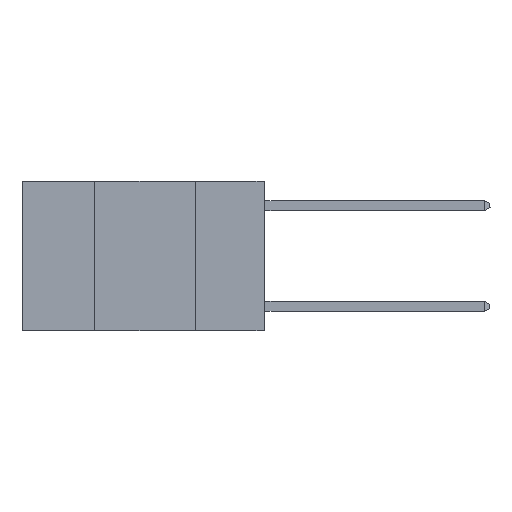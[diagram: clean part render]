
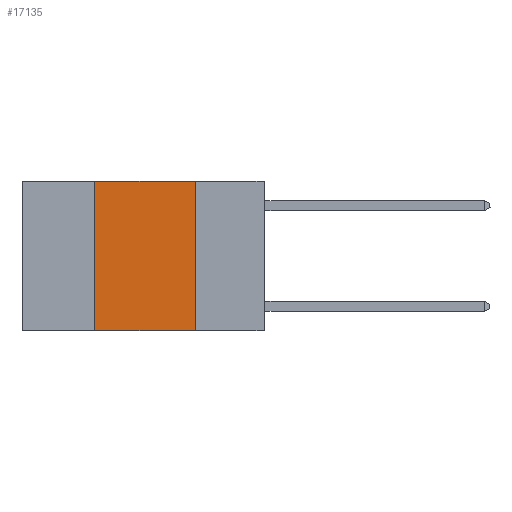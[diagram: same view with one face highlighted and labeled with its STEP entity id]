
A CAD part, left-side view. The second image highlights one B-rep face of the part: STEP entity #17135.
In plain terms, the highlighted planar face has unit normal (-1, 0, 0).
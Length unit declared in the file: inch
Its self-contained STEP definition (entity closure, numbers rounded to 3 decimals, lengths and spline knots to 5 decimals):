
#3728 = VECTOR ( 'NONE', #23854, 39.37008 ) ;
#3889 = LINE ( 'NONE', #4177, #15653 ) ;
#4177 = CARTESIAN_POINT ( 'NONE',  ( 0., 0.17, 0. ) ) ;
#4982 = VECTOR ( 'NONE', #8364, 39.37008 ) ;
#5128 = CARTESIAN_POINT ( 'NONE',  ( 0., 0.6, 0. ) ) ;
#6012 = CARTESIAN_POINT ( 'NONE',  ( 0., 0.6, -0.37 ) ) ;
#6512 = DIRECTION ( 'NONE',  ( 0., 0., -1. ) ) ;
#6677 = CARTESIAN_POINT ( 'NONE',  ( 0., 0.42, 0. ) ) ;
#8065 = DIRECTION ( 'NONE',  ( 1., 0., 0. ) ) ;
#8364 = DIRECTION ( 'NONE',  ( 0., -1., 0. ) ) ;
#8376 = EDGE_LOOP ( 'NONE', ( #15675, #22014, #15089, #15816 ) ) ;
#8590 = DIRECTION ( 'NONE',  ( 0., 0., 1. ) ) ;
#9260 = EDGE_CURVE ( 'NONE', #24364, #10238, #3889, .T. ) ;
#10238 = VERTEX_POINT ( 'NONE', #14322 ) ;
#13587 = EDGE_CURVE ( 'NONE', #28700, #24364, #23144, .T. ) ;
#14322 = CARTESIAN_POINT ( 'NONE',  ( 0., 0.17, -0.37 ) ) ;
#15089 = ORIENTED_EDGE ( 'NONE', *, *, #20933, .F. ) ;
#15090 = CARTESIAN_POINT ( 'NONE',  ( 0., 0.6, 0. ) ) ;
#15246 = LINE ( 'NONE', #17965, #26885 ) ;
#15653 = VECTOR ( 'NONE', #6512, 39.37008 ) ;
#15675 = ORIENTED_EDGE ( 'NONE', *, *, #9260, .F. ) ;
#15816 = ORIENTED_EDGE ( 'NONE', *, *, #25474, .T. ) ;
#16163 = CARTESIAN_POINT ( 'NONE',  ( 0., 0.17, 0. ) ) ;
#16275 = AXIS2_PLACEMENT_3D ( 'NONE', #15090, #8065, #24436 ) ;
#16429 = CARTESIAN_POINT ( 'NONE',  ( 0., 0.42, -0.37 ) ) ;
#16813 = VERTEX_POINT ( 'NONE', #16429 ) ;
#17135 = ADVANCED_FACE ( 'NONE', ( #17694 ), #19806, .F. ) ;
#17484 = LINE ( 'NONE', #6012, #4982 ) ;
#17694 = FACE_OUTER_BOUND ( 'NONE', #8376, .T. ) ;
#17965 = CARTESIAN_POINT ( 'NONE',  ( 0., 0.42, 0. ) ) ;
#19806 = PLANE ( 'NONE',  #16275 ) ;
#20933 = EDGE_CURVE ( 'NONE', #16813, #28700, #15246, .T. ) ;
#22014 = ORIENTED_EDGE ( 'NONE', *, *, #13587, .F. ) ;
#23144 = LINE ( 'NONE', #5128, #3728 ) ;
#23854 = DIRECTION ( 'NONE',  ( 0., -1., 0. ) ) ;
#24364 = VERTEX_POINT ( 'NONE', #16163 ) ;
#24436 = DIRECTION ( 'NONE',  ( 0., 0., -1. ) ) ;
#25474 = EDGE_CURVE ( 'NONE', #16813, #10238, #17484, .T. ) ;
#26885 = VECTOR ( 'NONE', #8590, 39.37008 ) ;
#28700 = VERTEX_POINT ( 'NONE', #6677 ) ;
